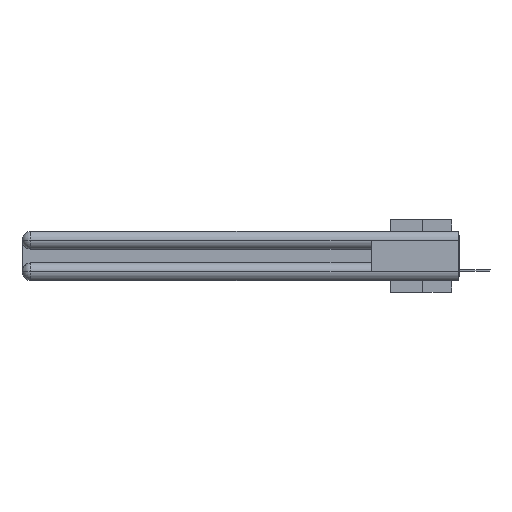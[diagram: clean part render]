
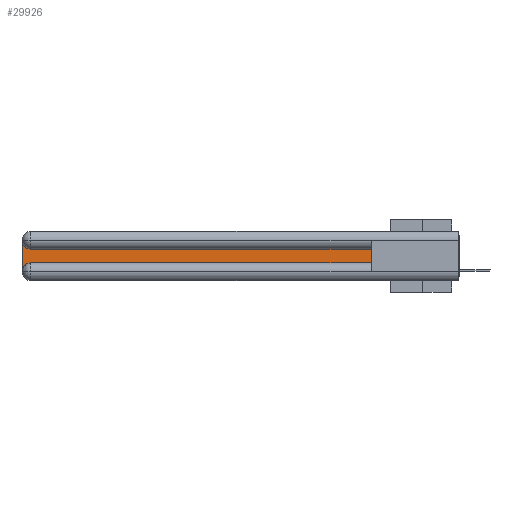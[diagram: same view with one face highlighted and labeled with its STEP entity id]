
A CAD part, left-side view. The second image highlights one B-rep face of the part: STEP entity #29926.
In plain terms, the highlighted planar face has unit normal (-1, 0, 0).
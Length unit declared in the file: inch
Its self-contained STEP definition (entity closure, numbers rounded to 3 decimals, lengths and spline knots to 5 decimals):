
#409 = DIRECTION ( 'NONE',  ( 0., 0., -1. ) ) ;
#733 = CARTESIAN_POINT ( 'NONE',  ( 0.075, 3., -0.1225 ) ) ;
#983 = EDGE_CURVE ( 'NONE', #29573, #9560, #11009, .T. ) ;
#2443 = LINE ( 'NONE', #16109, #23571 ) ;
#2937 = DIRECTION ( 'NONE',  ( 1., 0., 0. ) ) ;
#3515 = PLANE ( 'NONE',  #23626 ) ;
#4475 = CARTESIAN_POINT ( 'NONE',  ( 0.075, 3., -0.0625 ) ) ;
#4477 = CARTESIAN_POINT ( 'NONE',  ( 0.075, 0.6, -0.2175 ) ) ;
#5756 = DIRECTION ( 'NONE',  ( 0., 0., -1. ) ) ;
#5949 = VECTOR ( 'NONE', #10523, 39.37008 ) ;
#6859 = ORIENTED_EDGE ( 'NONE', *, *, #20636, .T. ) ;
#7187 = CARTESIAN_POINT ( 'NONE',  ( 0.075, 0.6, -0.2175 ) ) ;
#8127 = ORIENTED_EDGE ( 'NONE', *, *, #13498, .T. ) ;
#8445 = AXIS2_PLACEMENT_3D ( 'NONE', #35482, #2937, #5756 ) ;
#8636 = DIRECTION ( 'NONE',  ( 1., 0., 0. ) ) ;
#8642 = AXIS2_PLACEMENT_3D ( 'NONE', #26169, #25928, #34341 ) ;
#9560 = VERTEX_POINT ( 'NONE', #20114 ) ;
#10512 = ORIENTED_EDGE ( 'NONE', *, *, #983, .T. ) ;
#10523 = DIRECTION ( 'NONE',  ( 0., 0., 1. ) ) ;
#10612 = DIRECTION ( 'NONE',  ( 0., 1., 0. ) ) ;
#10769 = VERTEX_POINT ( 'NONE', #20759 ) ;
#10876 = VECTOR ( 'NONE', #409, 39.37008 ) ;
#11009 = CIRCLE ( 'NONE', #8642, 0.06 ) ;
#11270 = VERTEX_POINT ( 'NONE', #4475 ) ;
#11430 = CARTESIAN_POINT ( 'NONE',  ( 0.075, 3., -0.2175 ) ) ;
#11732 = EDGE_CURVE ( 'NONE', #10769, #22382, #2443, .T. ) ;
#13498 = EDGE_CURVE ( 'NONE', #9560, #27884, #23511, .T. ) ;
#15530 = ORIENTED_EDGE ( 'NONE', *, *, #11732, .T. ) ;
#15889 = CIRCLE ( 'NONE', #8445, 0.06 ) ;
#16109 = CARTESIAN_POINT ( 'NONE',  ( 0.075, 0.6, -0.1225 ) ) ;
#16182 = CARTESIAN_POINT ( 'NONE',  ( 0.075, 0.6, -0.2175 ) ) ;
#16716 = LINE ( 'NONE', #4477, #5949 ) ;
#16825 = LINE ( 'NONE', #11430, #10876 ) ;
#17917 = CARTESIAN_POINT ( 'NONE',  ( 0.075, 3., -0.2775 ) ) ;
#19171 = DIRECTION ( 'NONE',  ( 0., -1., 0. ) ) ;
#20114 = CARTESIAN_POINT ( 'NONE',  ( 0.075, 2.94, -0.2175 ) ) ;
#20636 = EDGE_CURVE ( 'NONE', #22382, #11270, #15889, .T. ) ;
#20759 = CARTESIAN_POINT ( 'NONE',  ( 0.075, 0.6, -0.1225 ) ) ;
#22382 = VERTEX_POINT ( 'NONE', #26711 ) ;
#22441 = DIRECTION ( 'NONE',  ( 0., 0., -1. ) ) ;
#23511 = LINE ( 'NONE', #16182, #23935 ) ;
#23571 = VECTOR ( 'NONE', #10612, 39.37008 ) ;
#23626 = AXIS2_PLACEMENT_3D ( 'NONE', #733, #8636, #22441 ) ;
#23935 = VECTOR ( 'NONE', #19171, 39.37008 ) ;
#24039 = EDGE_CURVE ( 'NONE', #27884, #10769, #16716, .T. ) ;
#25928 = DIRECTION ( 'NONE',  ( 1., 0., 0. ) ) ;
#26169 = CARTESIAN_POINT ( 'NONE',  ( 0.075, 2.94, -0.2775 ) ) ;
#26711 = CARTESIAN_POINT ( 'NONE',  ( 0.075, 2.94, -0.1225 ) ) ;
#27593 = ORIENTED_EDGE ( 'NONE', *, *, #34068, .T. ) ;
#27741 = ORIENTED_EDGE ( 'NONE', *, *, #24039, .T. ) ;
#27884 = VERTEX_POINT ( 'NONE', #7187 ) ;
#29573 = VERTEX_POINT ( 'NONE', #17917 ) ;
#29926 = ADVANCED_FACE ( 'NONE', ( #30961 ), #3515, .F. ) ;
#30961 = FACE_OUTER_BOUND ( 'NONE', #32908, .T. ) ;
#32908 = EDGE_LOOP ( 'NONE', ( #15530, #6859, #27593, #10512, #8127, #27741 ) ) ;
#34068 = EDGE_CURVE ( 'NONE', #11270, #29573, #16825, .T. ) ;
#34341 = DIRECTION ( 'NONE',  ( 0., 0., -1. ) ) ;
#35482 = CARTESIAN_POINT ( 'NONE',  ( 0.075, 2.94, -0.0625 ) ) ;
